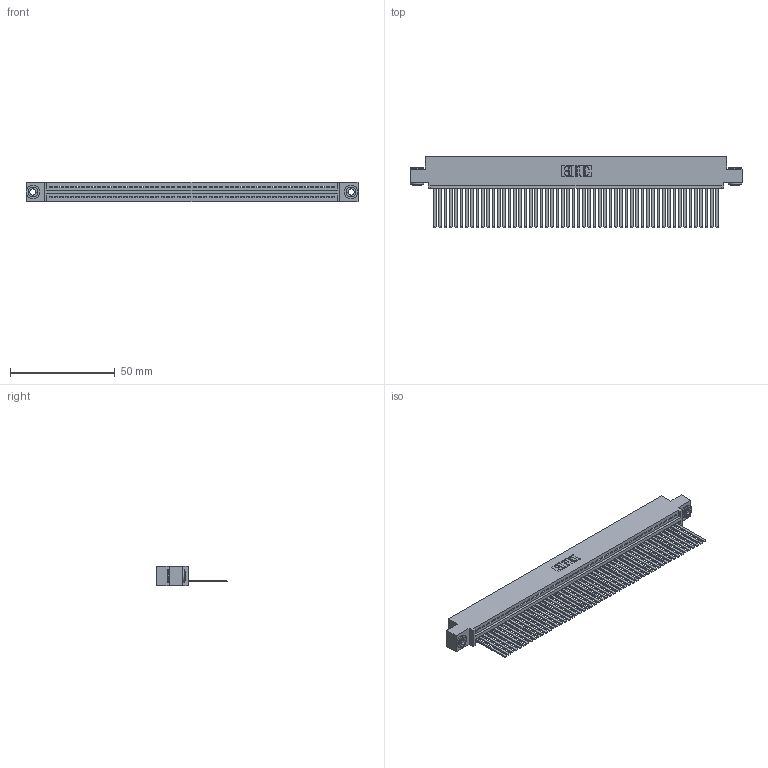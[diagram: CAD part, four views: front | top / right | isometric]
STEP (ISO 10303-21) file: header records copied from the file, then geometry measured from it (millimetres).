
FILE_DESCRIPTION (( 'STEP AP203' ), '1' );
FILE_NAME ('395-054-544-403.STEP', '2019-10-23T18:39:23', ( '' ), ( '' ), 'SwSTEP 2.0', 'SolidWorks 2016', '' );
FILE_SCHEMA (( 'CONFIG_CONTROL_DESIGN' ));
Length unit declared in the file: inch
Products named in the file (4): 395-054-544-403; 345 Part_0.110 Offset - 0.156 Dia-TH; 345-250-002_345-250-002-102; 345-292-001_345-293-144
Assembly tree (57 placements, depth 2):
  395-054-544-403
    345 Part_0.110 Offset - 0.156 Dia-TH
    345-292-001_345-293-144  x54
    345-250-002_345-250-002-102  x2
Bounding box: 158.37 x 33.96 x 9.4 mm (x, y, z)
Volume: 15711.8 mm3; surface area: 23216.5 mm2
Topology: 57 solids, 57 shells, 2976 faces, 8961 edges, 5898 vertices
Faces by surface type: plane 2038, cylinder 930, cone 8
Entity records: 39624 total; most frequent: CARTESIAN_POINT 6841, ORIENTED_EDGE 6822, DIRECTION 5985, EDGE_CURVE 3411, LINE 3043, VECTOR 3043, VERTEX_POINT 2270, AXIS2_PLACEMENT_3D 1471
